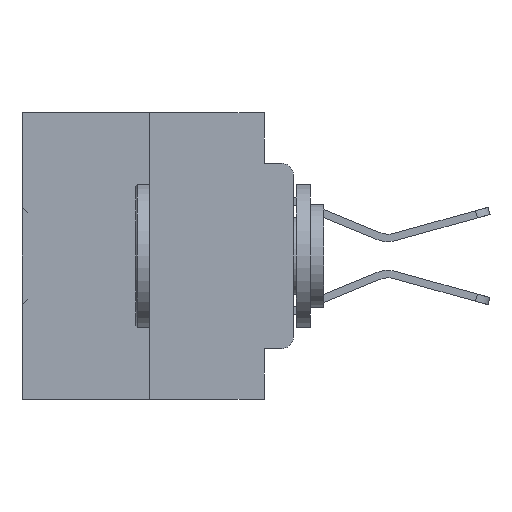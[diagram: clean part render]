
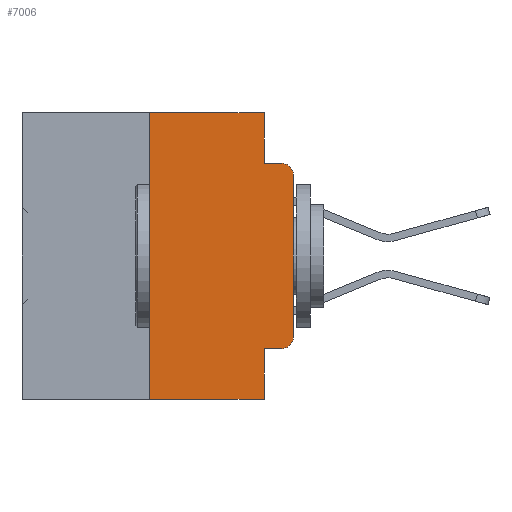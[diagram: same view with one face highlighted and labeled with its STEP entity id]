
A CAD part, left-side view. The second image highlights one B-rep face of the part: STEP entity #7006.
In plain terms, the highlighted planar face has unit normal (-1, 0, 0).
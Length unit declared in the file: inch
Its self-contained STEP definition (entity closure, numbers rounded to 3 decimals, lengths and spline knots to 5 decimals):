
#1232 = DIRECTION ( 'NONE',  ( -1., 0., 0. ) ) ;
#2001 = PLANE ( 'NONE',  #21662 ) ;
#2840 = ORIENTED_EDGE ( 'NONE', *, *, #24753, .F. ) ;
#2893 = VECTOR ( 'NONE', #13704, 39.37008 ) ;
#3614 = EDGE_CURVE ( 'NONE', #26094, #14352, #36527, .T. ) ;
#3734 = CARTESIAN_POINT ( 'NONE',  ( 0., 0., -0.3915 ) ) ;
#3738 = ORIENTED_EDGE ( 'NONE', *, *, #3614, .T. ) ;
#4179 = EDGE_LOOP ( 'NONE', ( #3738, #6575, #37902, #4274, #22372, #38389, #32332, #2840, #25737, #10480 ) ) ;
#4274 = ORIENTED_EDGE ( 'NONE', *, *, #28862, .F. ) ;
#4302 = VECTOR ( 'NONE', #25124, 39.37008 ) ;
#4492 = VECTOR ( 'NONE', #5450, 39.37008 ) ;
#5100 = DIRECTION ( 'NONE',  ( 1., 0., 0. ) ) ;
#5200 = LINE ( 'NONE', #33342, #21384 ) ;
#5450 = DIRECTION ( 'NONE',  ( 0., 0., -1. ) ) ;
#6575 = ORIENTED_EDGE ( 'NONE', *, *, #38858, .T. ) ;
#7006 = ADVANCED_FACE ( 'NONE', ( #22919 ), #2001, .F. ) ;
#7081 = DIRECTION ( 'NONE',  ( 0., -1., 0. ) ) ;
#7185 = CIRCLE ( 'NONE', #38840, 0.02 ) ;
#7582 = CARTESIAN_POINT ( 'NONE',  ( 0., 0.051, -0.4115 ) ) ;
#8230 = EDGE_CURVE ( 'NONE', #11581, #29714, #5200, .T. ) ;
#8500 = CARTESIAN_POINT ( 'NONE',  ( 0., 0.051, 0. ) ) ;
#9169 = DIRECTION ( 'NONE',  ( 0., -1., 0. ) ) ;
#10480 = ORIENTED_EDGE ( 'NONE', *, *, #18583, .T. ) ;
#11103 = CARTESIAN_POINT ( 'NONE',  ( 0., 0.473, 0. ) ) ;
#11581 = VERTEX_POINT ( 'NONE', #13945 ) ;
#11947 = LINE ( 'NONE', #34917, #2893 ) ;
#12742 = CARTESIAN_POINT ( 'NONE',  ( 0., 0.25, 0. ) ) ;
#13704 = DIRECTION ( 'NONE',  ( 0., 0., -1. ) ) ;
#13945 = CARTESIAN_POINT ( 'NONE',  ( 0., 0.25, -0.5 ) ) ;
#14125 = CARTESIAN_POINT ( 'NONE',  ( 0., 0.473, 0. ) ) ;
#14258 = DIRECTION ( 'NONE',  ( 0., -1., 0. ) ) ;
#14352 = VERTEX_POINT ( 'NONE', #22963 ) ;
#16508 = LINE ( 'NONE', #28384, #26568 ) ;
#16583 = CARTESIAN_POINT ( 'NONE',  ( 0., 0.02, -0.3915 ) ) ;
#16843 = VECTOR ( 'NONE', #17150, 39.37008 ) ;
#16909 = VERTEX_POINT ( 'NONE', #29658 ) ;
#17150 = DIRECTION ( 'NONE',  ( 0., -1., 0. ) ) ;
#18002 = VECTOR ( 'NONE', #14258, 39.37008 ) ;
#18583 = EDGE_CURVE ( 'NONE', #34264, #26094, #7185, .T. ) ;
#19077 = CARTESIAN_POINT ( 'NONE',  ( 0., 0.051, 0. ) ) ;
#19472 = CARTESIAN_POINT ( 'NONE',  ( 0., 0.02, -0.1085 ) ) ;
#19687 = DIRECTION ( 'NONE',  ( 0., 0., -1. ) ) ;
#20699 = EDGE_CURVE ( 'NONE', #21467, #34264, #16508, .T. ) ;
#21384 = VECTOR ( 'NONE', #9169, 39.37008 ) ;
#21467 = VERTEX_POINT ( 'NONE', #7582 ) ;
#21662 = AXIS2_PLACEMENT_3D ( 'NONE', #14125, #5100, #26383 ) ;
#22271 = EDGE_CURVE ( 'NONE', #29210, #34703, #24041, .T. ) ;
#22372 = ORIENTED_EDGE ( 'NONE', *, *, #22271, .F. ) ;
#22580 = DIRECTION ( 'NONE',  ( 0., 0., -1. ) ) ;
#22775 = CARTESIAN_POINT ( 'NONE',  ( 0., 0.02, -0.0885 ) ) ;
#22919 = FACE_OUTER_BOUND ( 'NONE', #4179, .T. ) ;
#22963 = CARTESIAN_POINT ( 'NONE',  ( 0., 0., -0.1085 ) ) ;
#23239 = LINE ( 'NONE', #28287, #32239 ) ;
#24041 = LINE ( 'NONE', #11103, #16843 ) ;
#24753 = EDGE_CURVE ( 'NONE', #21467, #29714, #11947, .T. ) ;
#25124 = DIRECTION ( 'NONE',  ( 0., 0., 1. ) ) ;
#25737 = ORIENTED_EDGE ( 'NONE', *, *, #20699, .T. ) ;
#26094 = VERTEX_POINT ( 'NONE', #3734 ) ;
#26173 = LINE ( 'NONE', #29441, #18002 ) ;
#26383 = DIRECTION ( 'NONE',  ( 0., 0., -1. ) ) ;
#26568 = VECTOR ( 'NONE', #7081, 39.37008 ) ;
#26803 = EDGE_CURVE ( 'NONE', #11581, #29210, #23239, .T. ) ;
#27458 = CARTESIAN_POINT ( 'NONE',  ( 0., 0.051, -0.5 ) ) ;
#27553 = AXIS2_PLACEMENT_3D ( 'NONE', #19472, #1232, #22580 ) ;
#28214 = VERTEX_POINT ( 'NONE', #22775 ) ;
#28287 = CARTESIAN_POINT ( 'NONE',  ( 0., 0.25, 0. ) ) ;
#28384 = CARTESIAN_POINT ( 'NONE',  ( 0., 0.051, -0.4115 ) ) ;
#28777 = LINE ( 'NONE', #8500, #4492 ) ;
#28862 = EDGE_CURVE ( 'NONE', #34703, #16909, #28777, .T. ) ;
#29210 = VERTEX_POINT ( 'NONE', #12742 ) ;
#29441 = CARTESIAN_POINT ( 'NONE',  ( 0., 0.051, -0.0885 ) ) ;
#29658 = CARTESIAN_POINT ( 'NONE',  ( 0., 0.051, -0.0885 ) ) ;
#29714 = VERTEX_POINT ( 'NONE', #27458 ) ;
#32239 = VECTOR ( 'NONE', #37183, 39.37008 ) ;
#32332 = ORIENTED_EDGE ( 'NONE', *, *, #8230, .T. ) ;
#32875 = EDGE_CURVE ( 'NONE', #16909, #28214, #26173, .T. ) ;
#33342 = CARTESIAN_POINT ( 'NONE',  ( 0., 0.473, -0.5 ) ) ;
#34264 = VERTEX_POINT ( 'NONE', #35866 ) ;
#34703 = VERTEX_POINT ( 'NONE', #19077 ) ;
#34917 = CARTESIAN_POINT ( 'NONE',  ( 0., 0.051, 0. ) ) ;
#35812 = CARTESIAN_POINT ( 'NONE',  ( 0., 0., 0. ) ) ;
#35866 = CARTESIAN_POINT ( 'NONE',  ( 0., 0.02, -0.4115 ) ) ;
#36527 = LINE ( 'NONE', #35812, #4302 ) ;
#37183 = DIRECTION ( 'NONE',  ( 0., 0., 1. ) ) ;
#37785 = DIRECTION ( 'NONE',  ( -1., 0., 0. ) ) ;
#37902 = ORIENTED_EDGE ( 'NONE', *, *, #32875, .F. ) ;
#38389 = ORIENTED_EDGE ( 'NONE', *, *, #26803, .F. ) ;
#38515 = CIRCLE ( 'NONE', #27553, 0.02 ) ;
#38840 = AXIS2_PLACEMENT_3D ( 'NONE', #16583, #37785, #19687 ) ;
#38858 = EDGE_CURVE ( 'NONE', #14352, #28214, #38515, .T. ) ;
